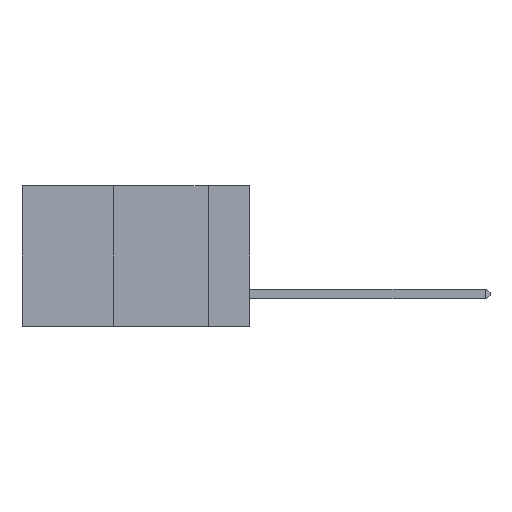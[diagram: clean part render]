
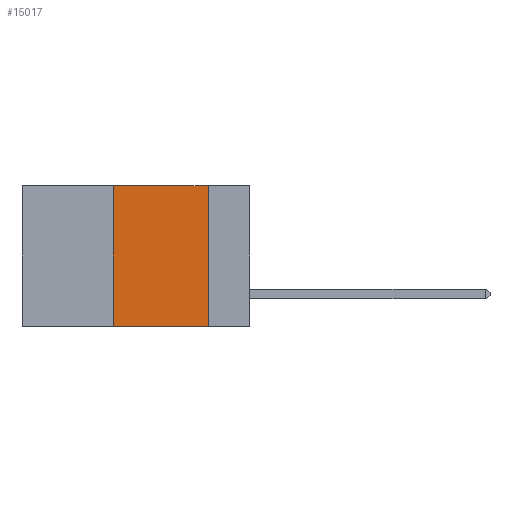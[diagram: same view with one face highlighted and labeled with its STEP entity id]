
A CAD part, left-side view. The second image highlights one B-rep face of the part: STEP entity #15017.
In plain terms, the highlighted planar face has unit normal (-1, 0, 0).
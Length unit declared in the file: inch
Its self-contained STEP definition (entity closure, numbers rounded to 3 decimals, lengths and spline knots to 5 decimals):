
#44 = VERTEX_POINT ( 'NONE', #15605 ) ;
#747 = CARTESIAN_POINT ( 'NONE',  ( 0., 0.6, 0. ) ) ;
#1321 = DIRECTION ( 'NONE',  ( 0., 0., 1. ) ) ;
#1453 = DIRECTION ( 'NONE',  ( 0., -1., 0. ) ) ;
#1846 = CARTESIAN_POINT ( 'NONE',  ( 0., 0.36, -0.37 ) ) ;
#2083 = VERTEX_POINT ( 'NONE', #4427 ) ;
#2177 = DIRECTION ( 'NONE',  ( 0., 0., -1. ) ) ;
#2336 = LINE ( 'NONE', #9257, #5921 ) ;
#2662 = DIRECTION ( 'NONE',  ( 0., 0., -1. ) ) ;
#4427 = CARTESIAN_POINT ( 'NONE',  ( 0., 0.11, 0. ) ) ;
#4478 = ORIENTED_EDGE ( 'NONE', *, *, #13357, .F. ) ;
#4634 = VERTEX_POINT ( 'NONE', #9898 ) ;
#4995 = LINE ( 'NONE', #16293, #9725 ) ;
#5899 = EDGE_CURVE ( 'NONE', #2083, #4634, #6511, .T. ) ;
#5921 = VECTOR ( 'NONE', #1321, 39.37008 ) ;
#5959 = CARTESIAN_POINT ( 'NONE',  ( 0., 0.11, 0. ) ) ;
#6133 = EDGE_CURVE ( 'NONE', #44, #2083, #15825, .T. ) ;
#6511 = LINE ( 'NONE', #5959, #6930 ) ;
#6548 = ORIENTED_EDGE ( 'NONE', *, *, #5899, .F. ) ;
#6930 = VECTOR ( 'NONE', #2662, 39.37008 ) ;
#7135 = FACE_OUTER_BOUND ( 'NONE', #13701, .T. ) ;
#8344 = DIRECTION ( 'NONE',  ( 0., -1., 0. ) ) ;
#8348 = CARTESIAN_POINT ( 'NONE',  ( 0., 0.6, 0. ) ) ;
#9257 = CARTESIAN_POINT ( 'NONE',  ( 0., 0.36, 0. ) ) ;
#9639 = VECTOR ( 'NONE', #8344, 39.37008 ) ;
#9725 = VECTOR ( 'NONE', #1453, 39.37008 ) ;
#9898 = CARTESIAN_POINT ( 'NONE',  ( 0., 0.11, -0.37 ) ) ;
#9964 = DIRECTION ( 'NONE',  ( 1., 0., 0. ) ) ;
#11518 = ORIENTED_EDGE ( 'NONE', *, *, #11965, .T. ) ;
#11965 = EDGE_CURVE ( 'NONE', #12714, #4634, #4995, .T. ) ;
#12714 = VERTEX_POINT ( 'NONE', #1846 ) ;
#13357 = EDGE_CURVE ( 'NONE', #12714, #44, #2336, .T. ) ;
#13570 = ORIENTED_EDGE ( 'NONE', *, *, #6133, .F. ) ;
#13701 = EDGE_LOOP ( 'NONE', ( #6548, #13570, #4478, #11518 ) ) ;
#14619 = PLANE ( 'NONE',  #15117 ) ;
#15017 = ADVANCED_FACE ( 'NONE', ( #7135 ), #14619, .F. ) ;
#15117 = AXIS2_PLACEMENT_3D ( 'NONE', #747, #9964, #2177 ) ;
#15605 = CARTESIAN_POINT ( 'NONE',  ( 0., 0.36, 0. ) ) ;
#15825 = LINE ( 'NONE', #8348, #9639 ) ;
#16293 = CARTESIAN_POINT ( 'NONE',  ( 0., 0.6, -0.37 ) ) ;
